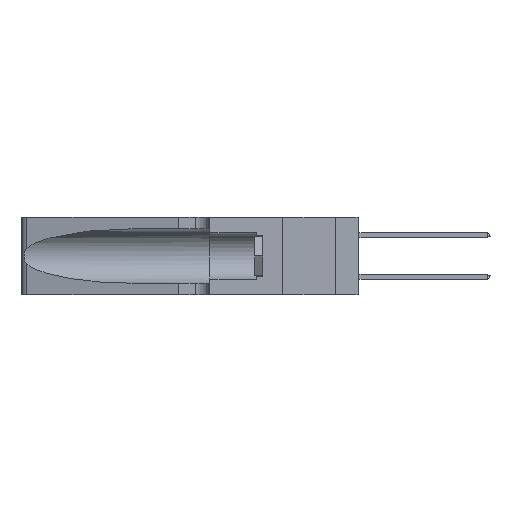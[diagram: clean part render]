
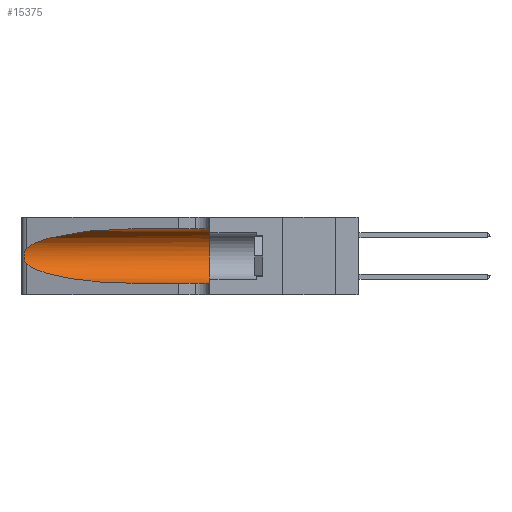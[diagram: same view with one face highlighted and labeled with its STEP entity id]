
A CAD part, left-side view. The second image highlights one B-rep face of the part: STEP entity #15375.
In plain terms, the highlighted cylindrical face has radius 3.308 mm (diameter 6.617 mm), a partial arc.
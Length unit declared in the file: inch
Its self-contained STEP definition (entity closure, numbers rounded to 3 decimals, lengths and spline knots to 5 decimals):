
#187 = VERTEX_POINT ( 'NONE', #7057 ) ;
#718 = CARTESIAN_POINT ( 'NONE',  ( 0.25487, 1.22718, 0.14631 ) ) ;
#823 = EDGE_CURVE ( 'NONE', #26397, #27774, #19731, .T. ) ;
#1201 = CARTESIAN_POINT ( 'NONE',  ( 0.1305, 0.72297, 0.05475 ) ) ;
#1710 = DIRECTION ( 'NONE',  ( 0., 0., -1. ) ) ;
#2060 = CARTESIAN_POINT ( 'NONE',  ( 0.25856, 1.23593, 0.16098 ) ) ;
#2301 = EDGE_CURVE ( 'NONE', #187, #2551, #31684, .T. ) ;
#2551 = VERTEX_POINT ( 'NONE', #38015 ) ;
#2704 = B_SPLINE_CURVE_WITH_KNOTS ( 'NONE', 3,
 ( #26385, #29352, #11201, #32334, #14305, #35335, #17382, #38285, #20458, #2060, #23505, #5148, #26513, #8258 ),
 .UNSPECIFIED., .F., .F.,
 ( 4, 2, 2, 2, 2, 2, 4 ),
 ( 0., 0.00027, 0.00053, 0.00107, 0.0016, 0.00187, 0.00214 ),
 .UNSPECIFIED. ) ;
#3779 = CARTESIAN_POINT ( 'NONE',  ( 0.1305, 0.72297, 0.31525 ) ) ;
#5038 = LINE ( 'NONE', #25792, #14205 ) ;
#5148 = CARTESIAN_POINT ( 'NONE',  ( 0.25639, 1.23186, 0.15144 ) ) ;
#6311 = CARTESIAN_POINT ( 'NONE',  ( 0.1305, 1.61858, 0.05475 ) ) ;
#6882 = CARTESIAN_POINT ( 'NONE',  ( 0.25487, 1.22718, 0.22369 ) ) ;
#7057 = CARTESIAN_POINT ( 'NONE',  ( 0.1305, 0.35, 0.31525 ) ) ;
#7347 = ORIENTED_EDGE ( 'NONE', *, *, #2301, .F. ) ;
#8258 = CARTESIAN_POINT ( 'NONE',  ( 0.25487, 1.22718, 0.14631 ) ) ;
#9866 = DIRECTION ( 'NONE',  ( 0., 1., 0. ) ) ;
#10147 = AXIS2_PLACEMENT_3D ( 'NONE', #28060, #9866, #31052 ) ;
#11201 = CARTESIAN_POINT ( 'NONE',  ( 0.25639, 1.23184, 0.21858 ) ) ;
#13457 = CARTESIAN_POINT ( 'NONE',  ( 0.2373, 1.15595, 0.08982 ) ) ;
#14205 = VECTOR ( 'NONE', #19691, 39.37008 ) ;
#14214 = EDGE_CURVE ( 'NONE', #21377, #30255, #32415, .T. ) ;
#14305 = CARTESIAN_POINT ( 'NONE',  ( 0.25854, 1.2359, 0.20912 ) ) ;
#15375 = ADVANCED_FACE ( 'NONE', ( #34575 ), #33649, .F. ) ;
#16016 = CARTESIAN_POINT ( 'NONE',  ( 0.2373, 1.15595, 0.28018 ) ) ;
#16129 = EDGE_CURVE ( 'NONE', #27774, #21377, #2704, .T. ) ;
#17382 = CARTESIAN_POINT ( 'NONE',  ( 0.26075, 1.23896, 0.19203 ) ) ;
#17871 = ORIENTED_EDGE ( 'NONE', *, *, #26533, .T. ) ;
#18704 = EDGE_LOOP ( 'NONE', ( #24945, #25455, #20696, #17871, #7347, #27053 ) ) ;
#19080 = CARTESIAN_POINT ( 'NONE',  ( 0.18966, 0.96281, 0.31525 ) ) ;
#19691 = DIRECTION ( 'NONE',  ( 0., -1., 0. ) ) ;
#19731 =( BOUNDED_CURVE ( )  B_SPLINE_CURVE ( 3, ( #3779, #19080, #16016, #6882 ),
 .UNSPECIFIED., .F., .T. ) 
 B_SPLINE_CURVE_WITH_KNOTS ( ( 4, 4 ),
 ( 1.5708, 2.84003 ),
 .UNSPECIFIED. ) 
 CURVE ( )  GEOMETRIC_REPRESENTATION_ITEM ( )  RATIONAL_B_SPLINE_CURVE ( ( 1., 0.87, 0.87, 1. ) ) 
 REPRESENTATION_ITEM ( '' )  );
#20097 = DIRECTION ( 'NONE',  ( 0., -1., 0. ) ) ;
#20198 = AXIS2_PLACEMENT_3D ( 'NONE', #34992, #20097, #1710 ) ;
#20458 = CARTESIAN_POINT ( 'NONE',  ( 0.26017, 1.23833, 0.17102 ) ) ;
#20696 = ORIENTED_EDGE ( 'NONE', *, *, #14214, .T. ) ;
#21377 = VERTEX_POINT ( 'NONE', #718 ) ;
#23465 = CARTESIAN_POINT ( 'NONE',  ( 0.1305, 0.72297, 0.05475 ) ) ;
#23505 = CARTESIAN_POINT ( 'NONE',  ( 0.25789, 1.23486, 0.15765 ) ) ;
#23976 = CARTESIAN_POINT ( 'NONE',  ( 0.1305, 0.72297, 0.31525 ) ) ;
#24945 = ORIENTED_EDGE ( 'NONE', *, *, #823, .T. ) ;
#25455 = ORIENTED_EDGE ( 'NONE', *, *, #16129, .T. ) ;
#25792 = CARTESIAN_POINT ( 'NONE',  ( 0.1305, 1.61858, 0.31525 ) ) ;
#26168 = CARTESIAN_POINT ( 'NONE',  ( 0.25487, 1.22718, 0.22369 ) ) ;
#26385 = CARTESIAN_POINT ( 'NONE',  ( 0.25487, 1.22718, 0.22369 ) ) ;
#26397 = VERTEX_POINT ( 'NONE', #23976 ) ;
#26513 = CARTESIAN_POINT ( 'NONE',  ( 0.25555, 1.22993, 0.14849 ) ) ;
#26520 = VECTOR ( 'NONE', #27631, 39.37008 ) ;
#26533 = EDGE_CURVE ( 'NONE', #30255, #2551, #33472, .T. ) ;
#27053 = ORIENTED_EDGE ( 'NONE', *, *, #30721, .F. ) ;
#27631 = DIRECTION ( 'NONE',  ( 0., -1., 0. ) ) ;
#27774 = VERTEX_POINT ( 'NONE', #26168 ) ;
#28060 = CARTESIAN_POINT ( 'NONE',  ( 0.1305, 0.35, 0.185 ) ) ;
#29352 = CARTESIAN_POINT ( 'NONE',  ( 0.25555, 1.22994, 0.2215 ) ) ;
#30255 = VERTEX_POINT ( 'NONE', #23465 ) ;
#30721 = EDGE_CURVE ( 'NONE', #26397, #187, #5038, .T. ) ;
#31052 = DIRECTION ( 'NONE',  ( 0., 0., 1. ) ) ;
#31502 = CARTESIAN_POINT ( 'NONE',  ( 0.18966, 0.96281, 0.05475 ) ) ;
#31684 = CIRCLE ( 'NONE', #10147, 0.13025 ) ;
#32334 = CARTESIAN_POINT ( 'NONE',  ( 0.25787, 1.23484, 0.2124 ) ) ;
#32415 =( BOUNDED_CURVE ( )  B_SPLINE_CURVE ( 3, ( #37449, #13457, #31502, #1201 ),
 .UNSPECIFIED., .F., .T. ) 
 B_SPLINE_CURVE_WITH_KNOTS ( ( 4, 4 ),
 ( 3.44316, 4.71239 ),
 .UNSPECIFIED. ) 
 CURVE ( )  GEOMETRIC_REPRESENTATION_ITEM ( )  RATIONAL_B_SPLINE_CURVE ( ( 1., 0.87, 0.87, 1. ) ) 
 REPRESENTATION_ITEM ( '' )  );
#33472 = LINE ( 'NONE', #6311, #26520 ) ;
#33649 = CYLINDRICAL_SURFACE ( 'NONE', #20198, 0.13025 ) ;
#34575 = FACE_OUTER_BOUND ( 'NONE', #18704, .T. ) ;
#34992 = CARTESIAN_POINT ( 'NONE',  ( 0.1305, 1.61858, 0.185 ) ) ;
#35335 = CARTESIAN_POINT ( 'NONE',  ( 0.26018, 1.23835, 0.19895 ) ) ;
#37449 = CARTESIAN_POINT ( 'NONE',  ( 0.25487, 1.22718, 0.14631 ) ) ;
#38015 = CARTESIAN_POINT ( 'NONE',  ( 0.1305, 0.35, 0.05475 ) ) ;
#38285 = CARTESIAN_POINT ( 'NONE',  ( 0.26075, 1.23896, 0.178 ) ) ;
